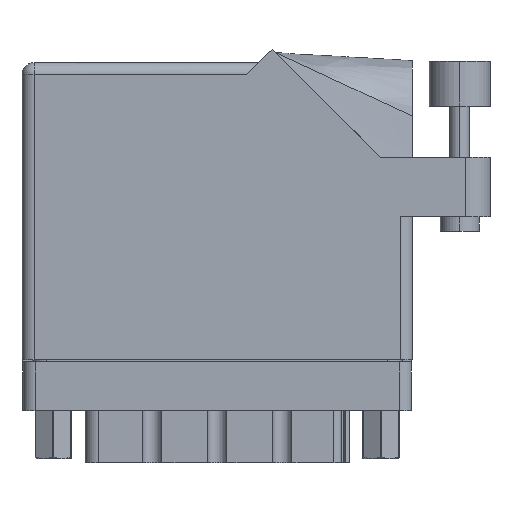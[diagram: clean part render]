
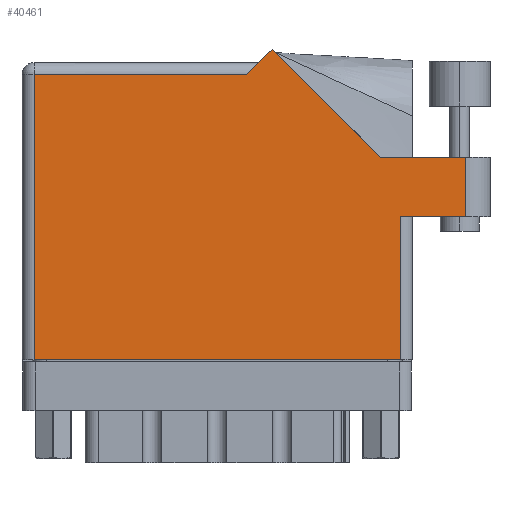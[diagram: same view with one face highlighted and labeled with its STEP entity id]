
A CAD part, front view. The second image highlights one B-rep face of the part: STEP entity #40461.
In plain terms, the highlighted face is planar.
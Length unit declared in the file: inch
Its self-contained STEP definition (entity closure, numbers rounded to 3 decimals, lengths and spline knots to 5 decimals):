
#105 = VECTOR ( 'NONE', #7402, 39.37008 ) ;
#480 = DIRECTION ( 'NONE',  ( 0., 1., 0. ) ) ;
#862 = LINE ( 'NONE', #11031, #9909 ) ;
#882 = CARTESIAN_POINT ( 'NONE',  ( 0.062, 1.468, 0. ) ) ;
#1825 = DIRECTION ( 'NONE',  ( -1., 0., 0. ) ) ;
#1978 = DIRECTION ( 'NONE',  ( -0.707, -0.707, 0. ) ) ;
#2034 = CARTESIAN_POINT ( 'NONE',  ( 1.84442, 1.044, 0. ) ) ;
#3284 = DIRECTION ( 'NONE',  ( 1., 0., 0. ) ) ;
#3336 = VERTEX_POINT ( 'NONE', #30651 ) ;
#3493 = ORIENTED_EDGE ( 'NONE', *, *, #15607, .T. ) ;
#4368 = EDGE_CURVE ( 'NONE', #48894, #27209, #39617, .T. ) ;
#5094 = CARTESIAN_POINT ( 'NONE',  ( 1.155, 1.468, 0. ) ) ;
#5695 = CARTESIAN_POINT ( 'NONE',  ( 1.217, 1.53, 0. ) ) ;
#7402 = DIRECTION ( 'NONE',  ( -1., 0., 0. ) ) ;
#7898 = LINE ( 'NONE', #7964, #30166 ) ;
#7900 = VERTEX_POINT ( 'NONE', #49425 ) ;
#7964 = CARTESIAN_POINT ( 'NONE',  ( 0.062, 0., 0. ) ) ;
#9553 = CARTESIAN_POINT ( 'NONE',  ( 2.285, 1.044, 0. ) ) ;
#9909 = VECTOR ( 'NONE', #3284, 39.37008 ) ;
#10093 = DIRECTION ( 'NONE',  ( 0., 1., 0. ) ) ;
#10999 = CARTESIAN_POINT ( 'NONE',  ( 1.948, 0., 0. ) ) ;
#11031 = CARTESIAN_POINT ( 'NONE',  ( 0., 0., 0. ) ) ;
#12794 = CARTESIAN_POINT ( 'NONE',  ( 2.01, 0.737, 0. ) ) ;
#15607 = EDGE_CURVE ( 'NONE', #40983, #3336, #25750, .T. ) ;
#15721 = VECTOR ( 'NONE', #24259, 39.37008 ) ;
#16476 = ORIENTED_EDGE ( 'NONE', *, *, #49596, .T. ) ;
#16787 = VERTEX_POINT ( 'NONE', #10999 ) ;
#17502 = DIRECTION ( 'NONE',  ( 0., 0., -1. ) ) ;
#19338 = LINE ( 'NONE', #12794, #15721 ) ;
#20580 = VERTEX_POINT ( 'NONE', #41990 ) ;
#20635 = EDGE_CURVE ( 'NONE', #27209, #20580, #7898, .T. ) ;
#20702 = PLANE ( 'NONE',  #22453 ) ;
#20880 = EDGE_CURVE ( 'NONE', #45716, #7900, #19338, .T. ) ;
#22412 = VERTEX_POINT ( 'NONE', #9553 ) ;
#22453 = AXIS2_PLACEMENT_3D ( 'NONE', #40579, #17502, #1825 ) ;
#24153 = ORIENTED_EDGE ( 'NONE', *, *, #20880, .T. ) ;
#24259 = DIRECTION ( 'NONE',  ( 1., 0., 0. ) ) ;
#24366 = CARTESIAN_POINT ( 'NONE',  ( 1.948, 0.737, 0. ) ) ;
#24702 = LINE ( 'NONE', #5695, #41553 ) ;
#25750 = LINE ( 'NONE', #2034, #32379 ) ;
#26289 = LINE ( 'NONE', #49318, #32933 ) ;
#27209 = VERTEX_POINT ( 'NONE', #882 ) ;
#28674 = DIRECTION ( 'NONE',  ( -0.707, 0.707, 0. ) ) ;
#29069 = LINE ( 'NONE', #45948, #105 ) ;
#29365 = VECTOR ( 'NONE', #33791, 39.37008 ) ;
#30166 = VECTOR ( 'NONE', #45852, 39.37008 ) ;
#30651 = CARTESIAN_POINT ( 'NONE',  ( 1.28771, 1.60071, 0. ) ) ;
#32047 = ORIENTED_EDGE ( 'NONE', *, *, #4368, .T. ) ;
#32244 = LINE ( 'NONE', #39588, #46108 ) ;
#32379 = VECTOR ( 'NONE', #28674, 39.37008 ) ;
#32933 = VECTOR ( 'NONE', #10093, 39.37008 ) ;
#33791 = DIRECTION ( 'NONE',  ( -1., 0., 0. ) ) ;
#35072 = ORIENTED_EDGE ( 'NONE', *, *, #46163, .T. ) ;
#35729 = ORIENTED_EDGE ( 'NONE', *, *, #41940, .T. ) ;
#36253 = ORIENTED_EDGE ( 'NONE', *, *, #45037, .T. ) ;
#36746 = ORIENTED_EDGE ( 'NONE', *, *, #20635, .T. ) ;
#39209 = CARTESIAN_POINT ( 'NONE',  ( 1.84442, 1.044, 0. ) ) ;
#39245 = ORIENTED_EDGE ( 'NONE', *, *, #47915, .T. ) ;
#39588 = CARTESIAN_POINT ( 'NONE',  ( 2.285, 1.044, 0. ) ) ;
#39617 = LINE ( 'NONE', #41398, #29365 ) ;
#40461 = ADVANCED_FACE ( 'NONE', ( #45585 ), #20702, .F. ) ;
#40579 = CARTESIAN_POINT ( 'NONE',  ( 0., 1.53, 0. ) ) ;
#40983 = VERTEX_POINT ( 'NONE', #39209 ) ;
#41398 = CARTESIAN_POINT ( 'NONE',  ( 0., 1.468, 0. ) ) ;
#41410 = EDGE_LOOP ( 'NONE', ( #24153, #35729, #39245, #3493, #16476, #32047, #36746, #35072, #36253 ) ) ;
#41553 = VECTOR ( 'NONE', #1978, 39.37008 ) ;
#41940 = EDGE_CURVE ( 'NONE', #7900, #22412, #32244, .T. ) ;
#41990 = CARTESIAN_POINT ( 'NONE',  ( 0.062, 0., 0. ) ) ;
#45037 = EDGE_CURVE ( 'NONE', #16787, #45716, #26289, .T. ) ;
#45585 = FACE_OUTER_BOUND ( 'NONE', #41410, .T. ) ;
#45716 = VERTEX_POINT ( 'NONE', #24366 ) ;
#45852 = DIRECTION ( 'NONE',  ( 0., -1., 0. ) ) ;
#45948 = CARTESIAN_POINT ( 'NONE',  ( 2.41, 1.044, 0. ) ) ;
#46108 = VECTOR ( 'NONE', #480, 39.37008 ) ;
#46163 = EDGE_CURVE ( 'NONE', #20580, #16787, #862, .T. ) ;
#47915 = EDGE_CURVE ( 'NONE', #22412, #40983, #29069, .T. ) ;
#48894 = VERTEX_POINT ( 'NONE', #5094 ) ;
#49318 = CARTESIAN_POINT ( 'NONE',  ( 1.948, 0.737, 0. ) ) ;
#49425 = CARTESIAN_POINT ( 'NONE',  ( 2.285, 0.737, 0. ) ) ;
#49596 = EDGE_CURVE ( 'NONE', #3336, #48894, #24702, .T. ) ;
